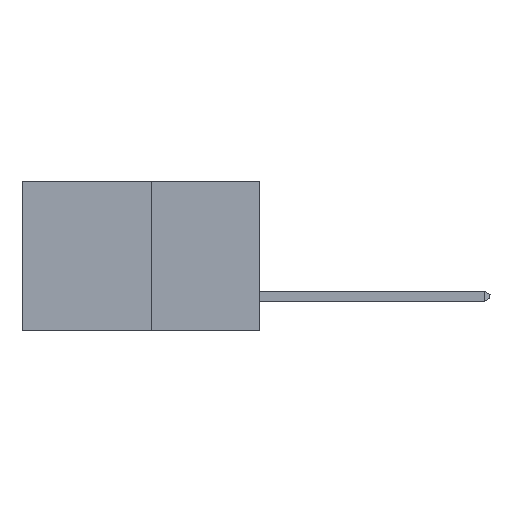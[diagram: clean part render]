
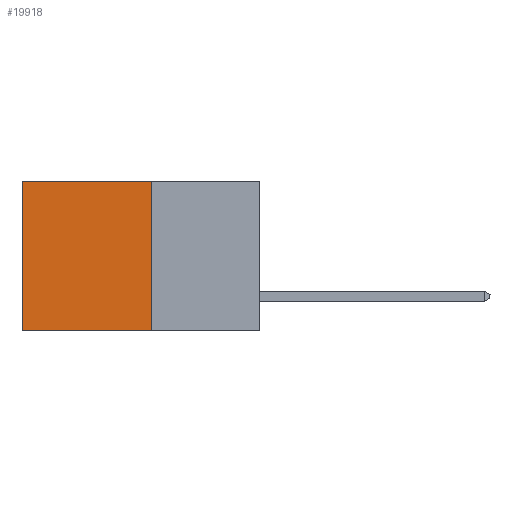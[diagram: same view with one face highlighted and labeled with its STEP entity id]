
A CAD part, left-side view. The second image highlights one B-rep face of the part: STEP entity #19918.
In plain terms, the highlighted planar face has unit normal (-1, 0, 0).
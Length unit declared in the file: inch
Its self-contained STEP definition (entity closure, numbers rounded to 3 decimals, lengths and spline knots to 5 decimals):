
#493 = VERTEX_POINT ( 'NONE', #10577 ) ;
#2551 = ORIENTED_EDGE ( 'NONE', *, *, #20815, .F. ) ;
#2816 = VECTOR ( 'NONE', #17642, 39.37008 ) ;
#3047 = PLANE ( 'NONE',  #21926 ) ;
#3278 = ORIENTED_EDGE ( 'NONE', *, *, #17416, .T. ) ;
#4348 = FACE_OUTER_BOUND ( 'NONE', #12107, .T. ) ;
#5652 = LINE ( 'NONE', #22995, #29408 ) ;
#6106 = CARTESIAN_POINT ( 'NONE',  ( 0.277, 0.27, -0.37 ) ) ;
#7761 = EDGE_CURVE ( 'NONE', #13538, #27839, #23488, .T. ) ;
#9098 = LINE ( 'NONE', #6106, #2816 ) ;
#10577 = CARTESIAN_POINT ( 'NONE',  ( 0.277, 0.27, 0. ) ) ;
#12107 = EDGE_LOOP ( 'NONE', ( #17351, #28441, #2551, #3278 ) ) ;
#12390 = CARTESIAN_POINT ( 'NONE',  ( 0.277, 0.27, -0.37 ) ) ;
#12495 = CARTESIAN_POINT ( 'NONE',  ( 0.277, 0.27, -0.37 ) ) ;
#12564 = DIRECTION ( 'NONE',  ( 0., 1., 0. ) ) ;
#12786 = CARTESIAN_POINT ( 'NONE',  ( 0.277, 0.59, -0.37 ) ) ;
#13538 = VERTEX_POINT ( 'NONE', #25504 ) ;
#14801 = DIRECTION ( 'NONE',  ( 0., 0., -1. ) ) ;
#15499 = CARTESIAN_POINT ( 'NONE',  ( 0.277, 0.59, 0. ) ) ;
#17351 = ORIENTED_EDGE ( 'NONE', *, *, #21649, .T. ) ;
#17416 = EDGE_CURVE ( 'NONE', #493, #18130, #22291, .T. ) ;
#17642 = DIRECTION ( 'NONE',  ( 0., 0., -1. ) ) ;
#18130 = VERTEX_POINT ( 'NONE', #15499 ) ;
#18494 = DIRECTION ( 'NONE',  ( 0., 0., -1. ) ) ;
#19918 = ADVANCED_FACE ( 'NONE', ( #4348 ), #3047, .F. ) ;
#19971 = CARTESIAN_POINT ( 'NONE',  ( 0.277, 0.27, 0. ) ) ;
#20815 = EDGE_CURVE ( 'NONE', #493, #13538, #9098, .T. ) ;
#21649 = EDGE_CURVE ( 'NONE', #18130, #27839, #5652, .T. ) ;
#21926 = AXIS2_PLACEMENT_3D ( 'NONE', #12495, #28490, #14801 ) ;
#22253 = DIRECTION ( 'NONE',  ( 0., 1., 0. ) ) ;
#22291 = LINE ( 'NONE', #19971, #27654 ) ;
#22995 = CARTESIAN_POINT ( 'NONE',  ( 0.277, 0.59, -0.37 ) ) ;
#23488 = LINE ( 'NONE', #12390, #24206 ) ;
#24206 = VECTOR ( 'NONE', #12564, 39.37008 ) ;
#25504 = CARTESIAN_POINT ( 'NONE',  ( 0.277, 0.27, -0.37 ) ) ;
#27654 = VECTOR ( 'NONE', #22253, 39.37008 ) ;
#27839 = VERTEX_POINT ( 'NONE', #12786 ) ;
#28441 = ORIENTED_EDGE ( 'NONE', *, *, #7761, .F. ) ;
#28490 = DIRECTION ( 'NONE',  ( 1., 0., 0. ) ) ;
#29408 = VECTOR ( 'NONE', #18494, 39.37008 ) ;
